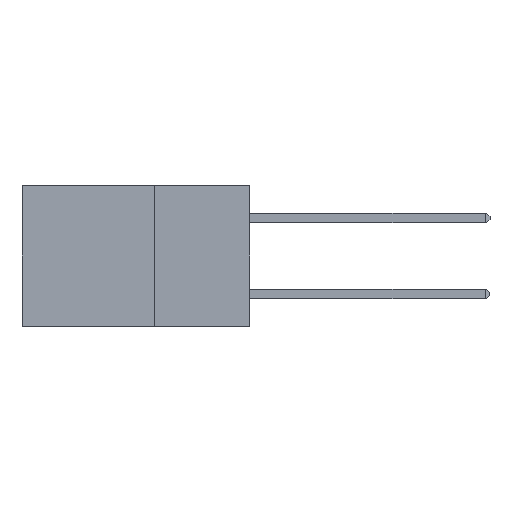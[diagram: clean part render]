
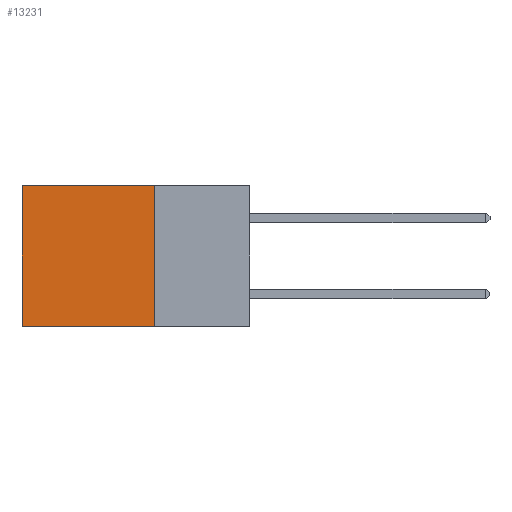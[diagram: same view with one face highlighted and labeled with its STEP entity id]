
A CAD part, left-side view. The second image highlights one B-rep face of the part: STEP entity #13231.
In plain terms, the highlighted planar face has unit normal (-1, 0, 0).
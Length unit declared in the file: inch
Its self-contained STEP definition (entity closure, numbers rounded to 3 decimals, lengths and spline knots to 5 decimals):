
#241 = EDGE_CURVE ( 'NONE', #9483, #11415, #4751, .T. ) ;
#270 = CARTESIAN_POINT ( 'NONE',  ( 0.2875, 0.25, 0. ) ) ;
#583 = PLANE ( 'NONE',  #15552 ) ;
#1264 = EDGE_LOOP ( 'NONE', ( #4533, #5435, #5497, #6586 ) ) ;
#1566 = VERTEX_POINT ( 'NONE', #1906 ) ;
#1636 = CARTESIAN_POINT ( 'NONE',  ( 0.2875, 0.25, 0. ) ) ;
#1691 = DIRECTION ( 'NONE',  ( 0., 0., -1. ) ) ;
#1825 = CARTESIAN_POINT ( 'NONE',  ( 0.2875, 0.25, 0. ) ) ;
#1841 = LINE ( 'NONE', #4887, #8550 ) ;
#1906 = CARTESIAN_POINT ( 'NONE',  ( 0.2875, 0.25, -0.37 ) ) ;
#3251 = DIRECTION ( 'NONE',  ( 0., 0., -1. ) ) ;
#3566 = FACE_OUTER_BOUND ( 'NONE', #1264, .T. ) ;
#3760 = CARTESIAN_POINT ( 'NONE',  ( 0.2875, 0.6, 0. ) ) ;
#4533 = ORIENTED_EDGE ( 'NONE', *, *, #4908, .T. ) ;
#4617 = DIRECTION ( 'NONE',  ( 0., 1., 0. ) ) ;
#4751 = LINE ( 'NONE', #270, #7305 ) ;
#4887 = CARTESIAN_POINT ( 'NONE',  ( 0.2875, 0.25, -0.37 ) ) ;
#4908 = EDGE_CURVE ( 'NONE', #11415, #12849, #6502, .T. ) ;
#5389 = EDGE_CURVE ( 'NONE', #1566, #12849, #1841, .T. ) ;
#5435 = ORIENTED_EDGE ( 'NONE', *, *, #5389, .F. ) ;
#5478 = EDGE_CURVE ( 'NONE', #9483, #1566, #9897, .T. ) ;
#5497 = ORIENTED_EDGE ( 'NONE', *, *, #5478, .F. ) ;
#6502 = LINE ( 'NONE', #8268, #12579 ) ;
#6586 = ORIENTED_EDGE ( 'NONE', *, *, #241, .T. ) ;
#7305 = VECTOR ( 'NONE', #13296, 39.37008 ) ;
#8268 = CARTESIAN_POINT ( 'NONE',  ( 0.2875, 0.6, 0. ) ) ;
#8550 = VECTOR ( 'NONE', #4617, 39.37008 ) ;
#8604 = DIRECTION ( 'NONE',  ( 0., 0., -1. ) ) ;
#9483 = VERTEX_POINT ( 'NONE', #1825 ) ;
#9897 = LINE ( 'NONE', #1636, #12735 ) ;
#10692 = DIRECTION ( 'NONE',  ( 1., 0., 0. ) ) ;
#11415 = VERTEX_POINT ( 'NONE', #3760 ) ;
#12562 = CARTESIAN_POINT ( 'NONE',  ( 0.2875, 0.6, -0.37 ) ) ;
#12579 = VECTOR ( 'NONE', #8604, 39.37008 ) ;
#12735 = VECTOR ( 'NONE', #1691, 39.37008 ) ;
#12849 = VERTEX_POINT ( 'NONE', #12562 ) ;
#13231 = ADVANCED_FACE ( 'NONE', ( #3566 ), #583, .F. ) ;
#13296 = DIRECTION ( 'NONE',  ( 0., 1., 0. ) ) ;
#15517 = CARTESIAN_POINT ( 'NONE',  ( 0.2875, 0.25, 0. ) ) ;
#15552 = AXIS2_PLACEMENT_3D ( 'NONE', #15517, #10692, #3251 ) ;
